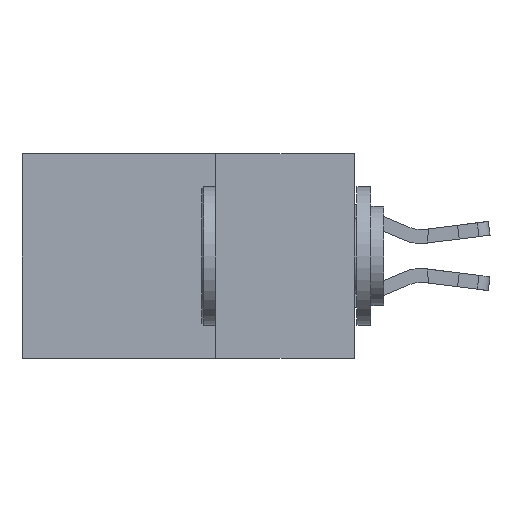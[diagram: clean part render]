
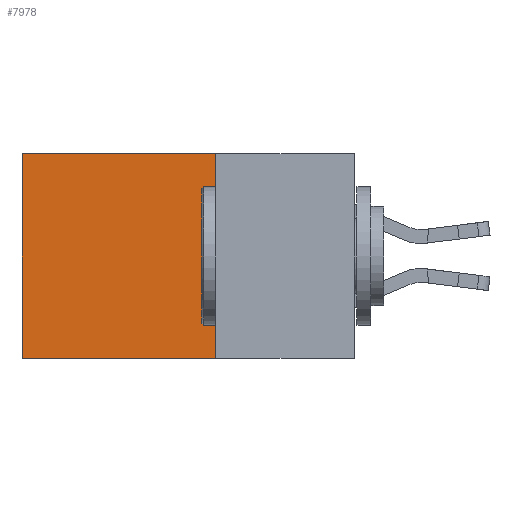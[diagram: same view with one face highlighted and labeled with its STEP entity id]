
A CAD part, left-side view. The second image highlights one B-rep face of the part: STEP entity #7978.
In plain terms, the highlighted planar face has unit normal (-1, 0, 0).
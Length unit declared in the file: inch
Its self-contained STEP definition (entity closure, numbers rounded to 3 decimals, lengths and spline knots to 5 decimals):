
#227 = ORIENTED_EDGE ( 'NONE', *, *, #2801, .T. ) ;
#1096 = VERTEX_POINT ( 'NONE', #8741 ) ;
#1446 = EDGE_CURVE ( 'NONE', #1925, #8376, #5541, .T. ) ;
#1565 = CARTESIAN_POINT ( 'NONE',  ( 0.2615, 0.25, -0.37 ) ) ;
#1663 = EDGE_CURVE ( 'NONE', #1096, #1925, #11839, .T. ) ;
#1791 = LINE ( 'NONE', #3935, #8060 ) ;
#1925 = VERTEX_POINT ( 'NONE', #1565 ) ;
#2112 = CARTESIAN_POINT ( 'NONE',  ( 0.2615, 0.25, -0.37 ) ) ;
#2169 = ORIENTED_EDGE ( 'NONE', *, *, #1446, .F. ) ;
#2382 = CARTESIAN_POINT ( 'NONE',  ( 0.2615, 0.25, 0. ) ) ;
#2489 = VERTEX_POINT ( 'NONE', #5564 ) ;
#2801 = EDGE_CURVE ( 'NONE', #1096, #2489, #10480, .T. ) ;
#3287 = VECTOR ( 'NONE', #12897, 39.37008 ) ;
#3735 = CARTESIAN_POINT ( 'NONE',  ( 0.2615, 0.6, -0.37 ) ) ;
#3935 = CARTESIAN_POINT ( 'NONE',  ( 0.2615, 0.6, -0.37 ) ) ;
#4964 = CARTESIAN_POINT ( 'NONE',  ( 0.2615, 0.25, -0.37 ) ) ;
#5221 = EDGE_LOOP ( 'NONE', ( #9131, #2169, #6911, #227 ) ) ;
#5541 = LINE ( 'NONE', #5677, #9608 ) ;
#5564 = CARTESIAN_POINT ( 'NONE',  ( 0.2615, 0.6, 0. ) ) ;
#5677 = CARTESIAN_POINT ( 'NONE',  ( 0.2615, 0.25, -0.37 ) ) ;
#5887 = DIRECTION ( 'NONE',  ( 0., 0., -1. ) ) ;
#6003 = DIRECTION ( 'NONE',  ( 0., 0., -1. ) ) ;
#6888 = DIRECTION ( 'NONE',  ( 1., 0., 0. ) ) ;
#6911 = ORIENTED_EDGE ( 'NONE', *, *, #1663, .F. ) ;
#7040 = VECTOR ( 'NONE', #9755, 39.37008 ) ;
#7978 = ADVANCED_FACE ( 'NONE', ( #11043 ), #8871, .F. ) ;
#8060 = VECTOR ( 'NONE', #6003, 39.37008 ) ;
#8376 = VERTEX_POINT ( 'NONE', #3735 ) ;
#8741 = CARTESIAN_POINT ( 'NONE',  ( 0.2615, 0.25, 0. ) ) ;
#8871 = PLANE ( 'NONE',  #11783 ) ;
#9131 = ORIENTED_EDGE ( 'NONE', *, *, #11799, .T. ) ;
#9608 = VECTOR ( 'NONE', #12631, 39.37008 ) ;
#9755 = DIRECTION ( 'NONE',  ( 0., 1., 0. ) ) ;
#10480 = LINE ( 'NONE', #2382, #7040 ) ;
#11043 = FACE_OUTER_BOUND ( 'NONE', #5221, .T. ) ;
#11783 = AXIS2_PLACEMENT_3D ( 'NONE', #4964, #6888, #5887 ) ;
#11799 = EDGE_CURVE ( 'NONE', #2489, #8376, #1791, .T. ) ;
#11839 = LINE ( 'NONE', #2112, #3287 ) ;
#12631 = DIRECTION ( 'NONE',  ( 0., 1., 0. ) ) ;
#12897 = DIRECTION ( 'NONE',  ( 0., 0., -1. ) ) ;
